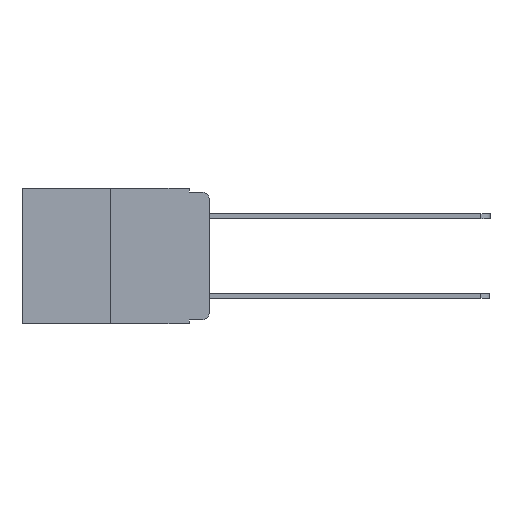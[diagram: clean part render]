
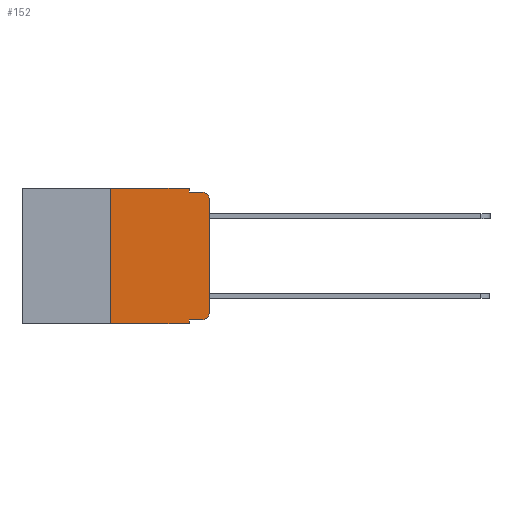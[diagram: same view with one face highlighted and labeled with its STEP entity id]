
A CAD part, left-side view. The second image highlights one B-rep face of the part: STEP entity #152.
In plain terms, the highlighted planar face has unit normal (-1, 0, 0).
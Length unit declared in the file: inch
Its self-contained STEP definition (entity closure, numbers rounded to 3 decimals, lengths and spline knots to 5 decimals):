
#152 = ADVANCED_FACE ( 'NONE', ( #3301 ), #8689, .F. ) ;
#497 = CARTESIAN_POINT ( 'NONE',  ( 0., 0.25, 0. ) ) ;
#526 = EDGE_LOOP ( 'NONE', ( #10523, #8508, #8278, #10073, #2949, #2971, #6787, #8522, #6575, #11593 ) ) ;
#605 = DIRECTION ( 'NONE',  ( -1., 0., 0. ) ) ;
#779 = EDGE_CURVE ( 'NONE', #14654, #5705, #16368, .T. ) ;
#809 = LINE ( 'NONE', #13065, #12199 ) ;
#952 = EDGE_CURVE ( 'NONE', #7981, #3307, #809, .T. ) ;
#1200 = VECTOR ( 'NONE', #3196, 39.37008 ) ;
#1906 = VECTOR ( 'NONE', #18468, 39.37008 ) ;
#2519 = CARTESIAN_POINT ( 'NONE',  ( 0., 0.051, -0.333 ) ) ;
#2949 = ORIENTED_EDGE ( 'NONE', *, *, #952, .F. ) ;
#2971 = ORIENTED_EDGE ( 'NONE', *, *, #15682, .F. ) ;
#3196 = DIRECTION ( 'NONE',  ( 0., 0., -1. ) ) ;
#3301 = FACE_OUTER_BOUND ( 'NONE', #526, .T. ) ;
#3307 = VERTEX_POINT ( 'NONE', #16970 ) ;
#3644 = LINE ( 'NONE', #4540, #11005 ) ;
#3769 = CARTESIAN_POINT ( 'NONE',  ( 0., 0., -0.03 ) ) ;
#3984 = CARTESIAN_POINT ( 'NONE',  ( 0., 0.051, -0.343 ) ) ;
#4155 = DIRECTION ( 'NONE',  ( 0., -1., 0. ) ) ;
#4540 = CARTESIAN_POINT ( 'NONE',  ( 0., 0.473, -0.343 ) ) ;
#4661 = VECTOR ( 'NONE', #10416, 39.37008 ) ;
#4828 = EDGE_CURVE ( 'NONE', #13051, #8187, #3644, .T. ) ;
#5705 = VERTEX_POINT ( 'NONE', #3769 ) ;
#5993 = LINE ( 'NONE', #6067, #1906 ) ;
#6067 = CARTESIAN_POINT ( 'NONE',  ( 0., 0.051, -0.01 ) ) ;
#6073 = DIRECTION ( 'NONE',  ( 0., -1., 0. ) ) ;
#6469 = CARTESIAN_POINT ( 'NONE',  ( 0., 0.02, -0.03 ) ) ;
#6575 = ORIENTED_EDGE ( 'NONE', *, *, #13898, .T. ) ;
#6731 = CARTESIAN_POINT ( 'NONE',  ( 0., 0., 0. ) ) ;
#6787 = ORIENTED_EDGE ( 'NONE', *, *, #4828, .T. ) ;
#6969 = CIRCLE ( 'NONE', #10082, 0.02 ) ;
#7227 = AXIS2_PLACEMENT_3D ( 'NONE', #6469, #16185, #7934 ) ;
#7241 = VERTEX_POINT ( 'NONE', #12002 ) ;
#7898 = VECTOR ( 'NONE', #17046, 39.37008 ) ;
#7934 = DIRECTION ( 'NONE',  ( 0., 0., -1. ) ) ;
#7981 = VERTEX_POINT ( 'NONE', #497 ) ;
#8187 = VERTEX_POINT ( 'NONE', #3984 ) ;
#8211 = CARTESIAN_POINT ( 'NONE',  ( 0., 0.02, -0.01 ) ) ;
#8278 = ORIENTED_EDGE ( 'NONE', *, *, #17442, .F. ) ;
#8508 = ORIENTED_EDGE ( 'NONE', *, *, #18328, .T. ) ;
#8522 = ORIENTED_EDGE ( 'NONE', *, *, #14800, .F. ) ;
#8689 = PLANE ( 'NONE',  #17043 ) ;
#8750 = VERTEX_POINT ( 'NONE', #8211 ) ;
#8906 = DIRECTION ( 'NONE',  ( 0., 0., -1. ) ) ;
#9032 = LINE ( 'NONE', #13137, #4661 ) ;
#9349 = CARTESIAN_POINT ( 'NONE',  ( 0., 0.02, -0.333 ) ) ;
#9620 = CARTESIAN_POINT ( 'NONE',  ( 0., 0.02, -0.313 ) ) ;
#9937 = VECTOR ( 'NONE', #15435, 39.37008 ) ;
#10073 = ORIENTED_EDGE ( 'NONE', *, *, #16578, .F. ) ;
#10082 = AXIS2_PLACEMENT_3D ( 'NONE', #9620, #605, #11074 ) ;
#10416 = DIRECTION ( 'NONE',  ( 0., 0., -1. ) ) ;
#10523 = ORIENTED_EDGE ( 'NONE', *, *, #779, .T. ) ;
#10688 = DIRECTION ( 'NONE',  ( 0., 0., 1. ) ) ;
#10823 = LINE ( 'NONE', #2519, #9937 ) ;
#11005 = VECTOR ( 'NONE', #6073, 39.37008 ) ;
#11074 = DIRECTION ( 'NONE',  ( 0., 0., -1. ) ) ;
#11403 = CIRCLE ( 'NONE', #7227, 0.02 ) ;
#11593 = ORIENTED_EDGE ( 'NONE', *, *, #13013, .T. ) ;
#11718 = LINE ( 'NONE', #14341, #7898 ) ;
#12002 = CARTESIAN_POINT ( 'NONE',  ( 0., 0.051, -0.01 ) ) ;
#12008 = CARTESIAN_POINT ( 'NONE',  ( 0., 0.051, 0. ) ) ;
#12199 = VECTOR ( 'NONE', #4155, 39.37008 ) ;
#12841 = VECTOR ( 'NONE', #10688, 39.37008 ) ;
#13013 = EDGE_CURVE ( 'NONE', #18350, #14654, #6969, .T. ) ;
#13051 = VERTEX_POINT ( 'NONE', #16487 ) ;
#13065 = CARTESIAN_POINT ( 'NONE',  ( 0., 0.473, 0. ) ) ;
#13137 = CARTESIAN_POINT ( 'NONE',  ( 0., 0.051, 0. ) ) ;
#13765 = CARTESIAN_POINT ( 'NONE',  ( 0., 0.473, 0. ) ) ;
#13898 = EDGE_CURVE ( 'NONE', #15680, #18350, #10823, .T. ) ;
#13962 = DIRECTION ( 'NONE',  ( 1., 0., 0. ) ) ;
#14341 = CARTESIAN_POINT ( 'NONE',  ( 0., 0.25, 0. ) ) ;
#14654 = VERTEX_POINT ( 'NONE', #16849 ) ;
#14800 = EDGE_CURVE ( 'NONE', #15680, #8187, #9032, .T. ) ;
#15435 = DIRECTION ( 'NONE',  ( 0., -1., 0. ) ) ;
#15680 = VERTEX_POINT ( 'NONE', #15728 ) ;
#15682 = EDGE_CURVE ( 'NONE', #13051, #7981, #11718, .T. ) ;
#15728 = CARTESIAN_POINT ( 'NONE',  ( 0., 0.051, -0.333 ) ) ;
#16185 = DIRECTION ( 'NONE',  ( -1., 0., 0. ) ) ;
#16368 = LINE ( 'NONE', #6731, #12841 ) ;
#16472 = LINE ( 'NONE', #12008, #1200 ) ;
#16487 = CARTESIAN_POINT ( 'NONE',  ( 0., 0.25, -0.343 ) ) ;
#16578 = EDGE_CURVE ( 'NONE', #3307, #7241, #16472, .T. ) ;
#16849 = CARTESIAN_POINT ( 'NONE',  ( 0., 0., -0.313 ) ) ;
#16970 = CARTESIAN_POINT ( 'NONE',  ( 0., 0.051, 0. ) ) ;
#17043 = AXIS2_PLACEMENT_3D ( 'NONE', #13765, #13962, #8906 ) ;
#17046 = DIRECTION ( 'NONE',  ( 0., 0., 1. ) ) ;
#17442 = EDGE_CURVE ( 'NONE', #7241, #8750, #5993, .T. ) ;
#18328 = EDGE_CURVE ( 'NONE', #5705, #8750, #11403, .T. ) ;
#18350 = VERTEX_POINT ( 'NONE', #9349 ) ;
#18468 = DIRECTION ( 'NONE',  ( 0., -1., 0. ) ) ;
